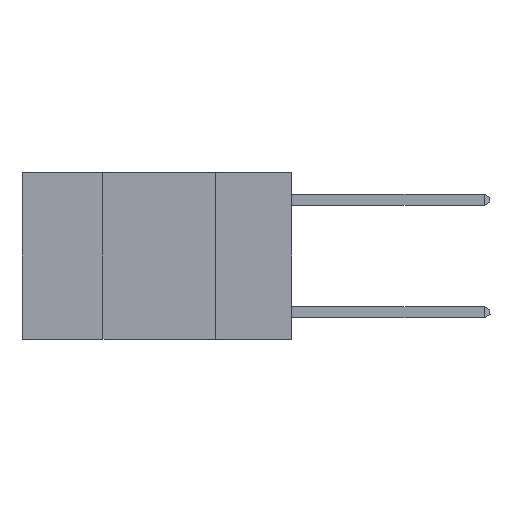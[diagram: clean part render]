
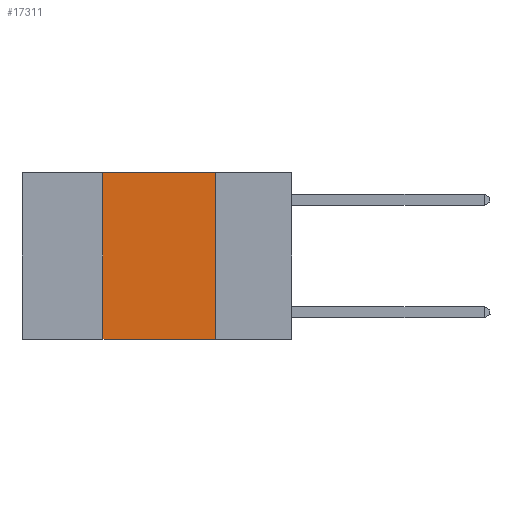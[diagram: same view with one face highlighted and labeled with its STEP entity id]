
A CAD part, left-side view. The second image highlights one B-rep face of the part: STEP entity #17311.
In plain terms, the highlighted planar face has unit normal (-1, 0, 0).
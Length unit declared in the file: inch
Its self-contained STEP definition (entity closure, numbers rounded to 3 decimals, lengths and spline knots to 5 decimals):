
#155 = ORIENTED_EDGE ( 'NONE', *, *, #13168, .F. ) ;
#2033 = EDGE_CURVE ( 'NONE', #17006, #13905, #15846, .T. ) ;
#2783 = PLANE ( 'NONE',  #6926 ) ;
#3036 = LINE ( 'NONE', #13692, #18004 ) ;
#3606 = LINE ( 'NONE', #17122, #9446 ) ;
#4796 = DIRECTION ( 'NONE',  ( 1., 0., 0. ) ) ;
#5445 = CARTESIAN_POINT ( 'NONE',  ( 0., 0.42, 0. ) ) ;
#5678 = EDGE_LOOP ( 'NONE', ( #20264, #155, #10537, #20870 ) ) ;
#6337 = CARTESIAN_POINT ( 'NONE',  ( 0., 0.42, 0. ) ) ;
#6926 = AXIS2_PLACEMENT_3D ( 'NONE', #16512, #4796, #18475 ) ;
#8966 = CARTESIAN_POINT ( 'NONE',  ( 0., 0.17, 0. ) ) ;
#9446 = VECTOR ( 'NONE', #24795, 39.37008 ) ;
#9730 = EDGE_CURVE ( 'NONE', #17006, #13884, #3036, .T. ) ;
#10537 = ORIENTED_EDGE ( 'NONE', *, *, #2033, .F. ) ;
#11226 = DIRECTION ( 'NONE',  ( 0., 0., -1. ) ) ;
#11320 = VECTOR ( 'NONE', #20055, 39.37008 ) ;
#12326 = VERTEX_POINT ( 'NONE', #8966 ) ;
#13168 = EDGE_CURVE ( 'NONE', #13905, #12326, #3606, .T. ) ;
#13692 = CARTESIAN_POINT ( 'NONE',  ( 0., 0.6, -0.37 ) ) ;
#13884 = VERTEX_POINT ( 'NONE', #17605 ) ;
#13905 = VERTEX_POINT ( 'NONE', #5445 ) ;
#14369 = EDGE_CURVE ( 'NONE', #12326, #13884, #22174, .T. ) ;
#15592 = DIRECTION ( 'NONE',  ( 0., -1., 0. ) ) ;
#15846 = LINE ( 'NONE', #6337, #11320 ) ;
#16371 = VECTOR ( 'NONE', #11226, 39.37008 ) ;
#16512 = CARTESIAN_POINT ( 'NONE',  ( 0., 0.6, 0. ) ) ;
#17006 = VERTEX_POINT ( 'NONE', #21552 ) ;
#17122 = CARTESIAN_POINT ( 'NONE',  ( 0., 0.6, 0. ) ) ;
#17311 = ADVANCED_FACE ( 'NONE', ( #18395 ), #2783, .F. ) ;
#17605 = CARTESIAN_POINT ( 'NONE',  ( 0., 0.17, -0.37 ) ) ;
#18004 = VECTOR ( 'NONE', #15592, 39.37008 ) ;
#18395 = FACE_OUTER_BOUND ( 'NONE', #5678, .T. ) ;
#18475 = DIRECTION ( 'NONE',  ( 0., 0., -1. ) ) ;
#20055 = DIRECTION ( 'NONE',  ( 0., 0., 1. ) ) ;
#20264 = ORIENTED_EDGE ( 'NONE', *, *, #14369, .F. ) ;
#20870 = ORIENTED_EDGE ( 'NONE', *, *, #9730, .T. ) ;
#21552 = CARTESIAN_POINT ( 'NONE',  ( 0., 0.42, -0.37 ) ) ;
#22174 = LINE ( 'NONE', #24743, #16371 ) ;
#24743 = CARTESIAN_POINT ( 'NONE',  ( 0., 0.17, 0. ) ) ;
#24795 = DIRECTION ( 'NONE',  ( 0., -1., 0. ) ) ;
